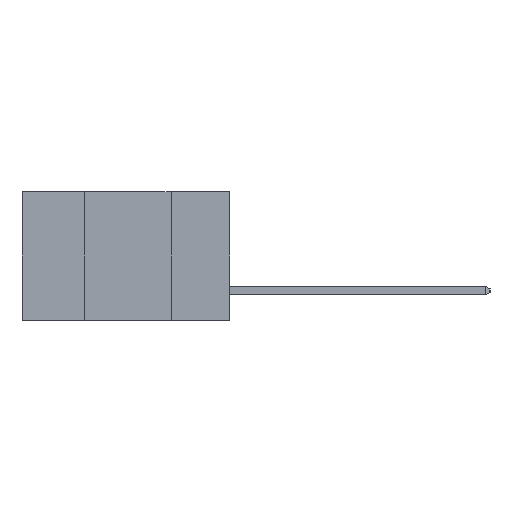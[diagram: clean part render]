
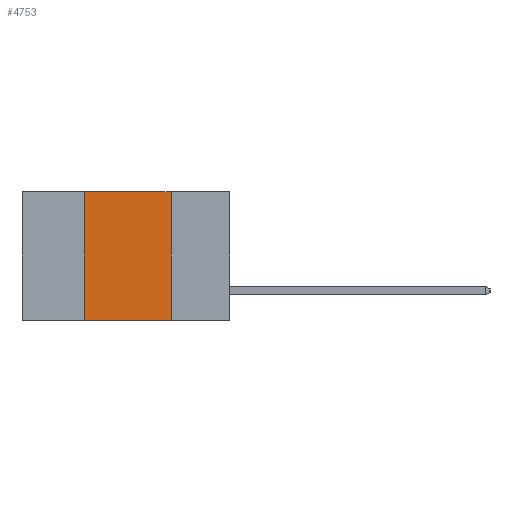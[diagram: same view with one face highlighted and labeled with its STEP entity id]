
A CAD part, left-side view. The second image highlights one B-rep face of the part: STEP entity #4753.
In plain terms, the highlighted planar face has unit normal (-1, 0, 0).
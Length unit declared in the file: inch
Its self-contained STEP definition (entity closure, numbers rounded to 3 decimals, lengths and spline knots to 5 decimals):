
#328 = PLANE ( 'NONE',  #5992 ) ;
#444 = VERTEX_POINT ( 'NONE', #14951 ) ;
#682 = LINE ( 'NONE', #12470, #7158 ) ;
#917 = CARTESIAN_POINT ( 'NONE',  ( 0., 0.17, -0.37 ) ) ;
#1666 = EDGE_CURVE ( 'NONE', #2605, #10649, #682, .T. ) ;
#1750 = ORIENTED_EDGE ( 'NONE', *, *, #1666, .F. ) ;
#2605 = VERTEX_POINT ( 'NONE', #11449 ) ;
#3031 = DIRECTION ( 'NONE',  ( 0., -1., 0. ) ) ;
#4549 = CARTESIAN_POINT ( 'NONE',  ( 0., 0.6, -0.37 ) ) ;
#4753 = ADVANCED_FACE ( 'NONE', ( #12248 ), #328, .F. ) ;
#5279 = CARTESIAN_POINT ( 'NONE',  ( 0., 0.17, 0. ) ) ;
#5547 = EDGE_LOOP ( 'NONE', ( #6256, #1750, #8643, #5648 ) ) ;
#5648 = ORIENTED_EDGE ( 'NONE', *, *, #7126, .T. ) ;
#5914 = DIRECTION ( 'NONE',  ( 0., 0., -1. ) ) ;
#5992 = AXIS2_PLACEMENT_3D ( 'NONE', #6023, #12672, #5914 ) ;
#6023 = CARTESIAN_POINT ( 'NONE',  ( 0., 0.6, 0. ) ) ;
#6256 = ORIENTED_EDGE ( 'NONE', *, *, #8826, .F. ) ;
#6394 = DIRECTION ( 'NONE',  ( 0., -1., 0. ) ) ;
#6880 = DIRECTION ( 'NONE',  ( 0., 0., 1. ) ) ;
#7126 = EDGE_CURVE ( 'NONE', #444, #14903, #12355, .T. ) ;
#7158 = VECTOR ( 'NONE', #6394, 39.37008 ) ;
#7980 = EDGE_CURVE ( 'NONE', #444, #2605, #8698, .T. ) ;
#8299 = VECTOR ( 'NONE', #6880, 39.37008 ) ;
#8643 = ORIENTED_EDGE ( 'NONE', *, *, #7980, .F. ) ;
#8698 = LINE ( 'NONE', #12099, #8299 ) ;
#8826 = EDGE_CURVE ( 'NONE', #10649, #14903, #16078, .T. ) ;
#9032 = DIRECTION ( 'NONE',  ( 0., 0., -1. ) ) ;
#10649 = VERTEX_POINT ( 'NONE', #11797 ) ;
#11449 = CARTESIAN_POINT ( 'NONE',  ( 0., 0.42, 0. ) ) ;
#11797 = CARTESIAN_POINT ( 'NONE',  ( 0., 0.17, 0. ) ) ;
#11957 = VECTOR ( 'NONE', #3031, 39.37008 ) ;
#12099 = CARTESIAN_POINT ( 'NONE',  ( 0., 0.42, 0. ) ) ;
#12248 = FACE_OUTER_BOUND ( 'NONE', #5547, .T. ) ;
#12355 = LINE ( 'NONE', #4549, #11957 ) ;
#12470 = CARTESIAN_POINT ( 'NONE',  ( 0., 0.6, 0. ) ) ;
#12672 = DIRECTION ( 'NONE',  ( 1., 0., 0. ) ) ;
#12722 = VECTOR ( 'NONE', #9032, 39.37008 ) ;
#14903 = VERTEX_POINT ( 'NONE', #917 ) ;
#14951 = CARTESIAN_POINT ( 'NONE',  ( 0., 0.42, -0.37 ) ) ;
#16078 = LINE ( 'NONE', #5279, #12722 ) ;
